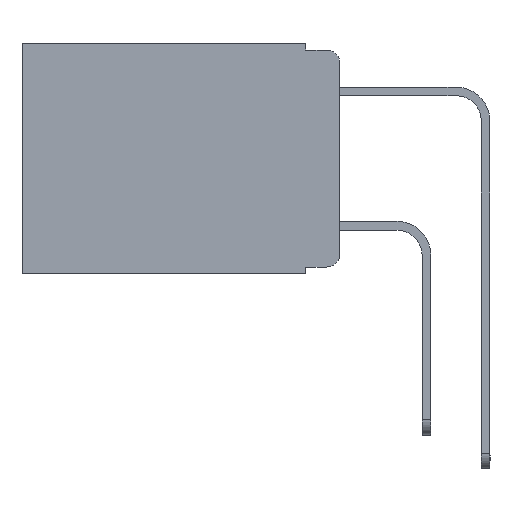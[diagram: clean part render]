
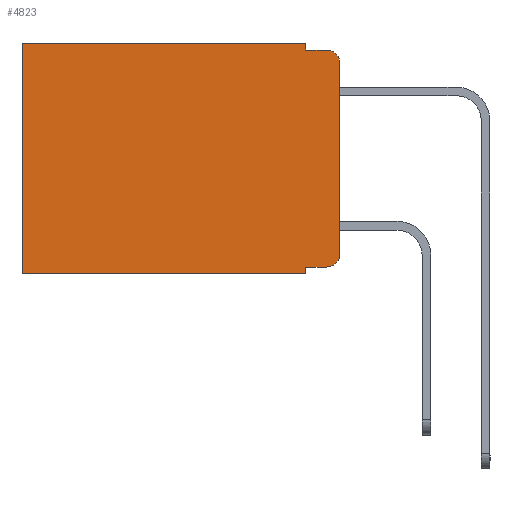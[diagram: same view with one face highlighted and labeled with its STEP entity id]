
A CAD part, left-side view. The second image highlights one B-rep face of the part: STEP entity #4823.
In plain terms, the highlighted planar face has unit normal (-1, 0, 0).
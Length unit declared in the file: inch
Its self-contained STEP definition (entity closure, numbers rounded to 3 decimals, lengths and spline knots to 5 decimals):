
#59 = ORIENTED_EDGE ( 'NONE', *, *, #6314, .F. ) ;
#996 = CARTESIAN_POINT ( 'NONE',  ( 0.298, 0.051, -0.333 ) ) ;
#1354 = EDGE_CURVE ( 'NONE', #11542, #20288, #14897, .T. ) ;
#1547 = DIRECTION ( 'NONE',  ( 1., 0., 0. ) ) ;
#1729 = VECTOR ( 'NONE', #17681, 39.37008 ) ;
#1819 = CARTESIAN_POINT ( 'NONE',  ( 0.298, 0., 0. ) ) ;
#2056 = LINE ( 'NONE', #6433, #13074 ) ;
#2120 = CARTESIAN_POINT ( 'NONE',  ( 0.298, 0.051, 0. ) ) ;
#2134 = DIRECTION ( 'NONE',  ( 0., 0., -1. ) ) ;
#2136 = CARTESIAN_POINT ( 'NONE',  ( 0.298, 0.051, -0.333 ) ) ;
#2709 = ORIENTED_EDGE ( 'NONE', *, *, #14870, .F. ) ;
#2943 = DIRECTION ( 'NONE',  ( -1., 0., 0. ) ) ;
#3644 = ORIENTED_EDGE ( 'NONE', *, *, #13271, .F. ) ;
#4561 = VERTEX_POINT ( 'NONE', #2136 ) ;
#4633 = ORIENTED_EDGE ( 'NONE', *, *, #1354, .T. ) ;
#4823 = ADVANCED_FACE ( 'NONE', ( #20280 ), #16604, .F. ) ;
#5040 = CIRCLE ( 'NONE', #22920, 0.02 ) ;
#5417 = CARTESIAN_POINT ( 'NONE',  ( 0.298, 0.051, 0. ) ) ;
#5519 = CARTESIAN_POINT ( 'NONE',  ( 0.298, 0.473, -0.343 ) ) ;
#5904 = VECTOR ( 'NONE', #26792, 39.37008 ) ;
#6314 = EDGE_CURVE ( 'NONE', #6345, #19972, #15251, .T. ) ;
#6345 = VERTEX_POINT ( 'NONE', #13186 ) ;
#6433 = CARTESIAN_POINT ( 'NONE',  ( 0.298, 0., 0. ) ) ;
#6496 = DIRECTION ( 'NONE',  ( 0., 0., -1. ) ) ;
#6515 = LINE ( 'NONE', #20582, #26492 ) ;
#6570 = CARTESIAN_POINT ( 'NONE',  ( 0.298, 0., -0.313 ) ) ;
#8101 = DIRECTION ( 'NONE',  ( 0., 0., -1. ) ) ;
#9087 = CARTESIAN_POINT ( 'NONE',  ( 0.298, 0.051, -0.01 ) ) ;
#9111 = CARTESIAN_POINT ( 'NONE',  ( 0.298, 0.02, -0.03 ) ) ;
#9128 = VECTOR ( 'NONE', #12824, 39.37008 ) ;
#9235 = VERTEX_POINT ( 'NONE', #26487 ) ;
#9357 = VECTOR ( 'NONE', #19869, 39.37008 ) ;
#9728 = VECTOR ( 'NONE', #11673, 39.37008 ) ;
#10088 = AXIS2_PLACEMENT_3D ( 'NONE', #1819, #1547, #8101 ) ;
#10370 = ORIENTED_EDGE ( 'NONE', *, *, #14620, .T. ) ;
#10512 = VERTEX_POINT ( 'NONE', #5417 ) ;
#11167 = CARTESIAN_POINT ( 'NONE',  ( 0.298, 0.473, 0. ) ) ;
#11542 = VERTEX_POINT ( 'NONE', #11167 ) ;
#11673 = DIRECTION ( 'NONE',  ( 0., 0., -1. ) ) ;
#12191 = CARTESIAN_POINT ( 'NONE',  ( 0.298, 0.02, -0.333 ) ) ;
#12503 = LINE ( 'NONE', #2120, #21305 ) ;
#12824 = DIRECTION ( 'NONE',  ( 0., 0., -1. ) ) ;
#13074 = VECTOR ( 'NONE', #25041, 39.37008 ) ;
#13186 = CARTESIAN_POINT ( 'NONE',  ( 0.298, 0.051, -0.01 ) ) ;
#13271 = EDGE_CURVE ( 'NONE', #10512, #6345, #12503, .T. ) ;
#14493 = VERTEX_POINT ( 'NONE', #12191 ) ;
#14620 = EDGE_CURVE ( 'NONE', #10512, #11542, #2056, .T. ) ;
#14870 = EDGE_CURVE ( 'NONE', #4561, #9235, #26395, .T. ) ;
#14897 = LINE ( 'NONE', #25414, #9128 ) ;
#14898 = CARTESIAN_POINT ( 'NONE',  ( 0.298, 0.02, -0.01 ) ) ;
#15251 = LINE ( 'NONE', #9087, #9357 ) ;
#15509 = EDGE_CURVE ( 'NONE', #14493, #24336, #5040, .T. ) ;
#16604 = PLANE ( 'NONE',  #10088 ) ;
#16821 = EDGE_CURVE ( 'NONE', #9235, #20288, #6515, .T. ) ;
#16909 = DIRECTION ( 'NONE',  ( -1., 0., 0. ) ) ;
#17528 = ORIENTED_EDGE ( 'NONE', *, *, #22072, .T. ) ;
#17681 = DIRECTION ( 'NONE',  ( 0., -1., 0. ) ) ;
#17815 = LINE ( 'NONE', #996, #1729 ) ;
#18314 = CARTESIAN_POINT ( 'NONE',  ( 0.298, 0.051, 0. ) ) ;
#18742 = ORIENTED_EDGE ( 'NONE', *, *, #21507, .T. ) ;
#19869 = DIRECTION ( 'NONE',  ( 0., -1., 0. ) ) ;
#19972 = VERTEX_POINT ( 'NONE', #14898 ) ;
#20280 = FACE_OUTER_BOUND ( 'NONE', #26678, .T. ) ;
#20288 = VERTEX_POINT ( 'NONE', #5519 ) ;
#20582 = CARTESIAN_POINT ( 'NONE',  ( 0.298, 0., -0.343 ) ) ;
#20673 = CARTESIAN_POINT ( 'NONE',  ( 0.298, 0., -0.03 ) ) ;
#20943 = ORIENTED_EDGE ( 'NONE', *, *, #16821, .F. ) ;
#21305 = VECTOR ( 'NONE', #6496, 39.37008 ) ;
#21507 = EDGE_CURVE ( 'NONE', #21712, #19972, #26205, .T. ) ;
#21712 = VERTEX_POINT ( 'NONE', #20673 ) ;
#21893 = ORIENTED_EDGE ( 'NONE', *, *, #15509, .T. ) ;
#22072 = EDGE_CURVE ( 'NONE', #4561, #14493, #17815, .T. ) ;
#22920 = AXIS2_PLACEMENT_3D ( 'NONE', #23059, #16909, #2134 ) ;
#23059 = CARTESIAN_POINT ( 'NONE',  ( 0.298, 0.02, -0.313 ) ) ;
#23755 = DIRECTION ( 'NONE',  ( 0., 0., -1. ) ) ;
#24014 = AXIS2_PLACEMENT_3D ( 'NONE', #9111, #2943, #23755 ) ;
#24336 = VERTEX_POINT ( 'NONE', #6570 ) ;
#24786 = CARTESIAN_POINT ( 'NONE',  ( 0.298, 0., 0. ) ) ;
#25036 = ORIENTED_EDGE ( 'NONE', *, *, #26623, .F. ) ;
#25041 = DIRECTION ( 'NONE',  ( 0., 1., 0. ) ) ;
#25109 = DIRECTION ( 'NONE',  ( 0., 1., 0. ) ) ;
#25414 = CARTESIAN_POINT ( 'NONE',  ( 0.298, 0.473, 0. ) ) ;
#26205 = CIRCLE ( 'NONE', #24014, 0.02 ) ;
#26395 = LINE ( 'NONE', #18314, #5904 ) ;
#26487 = CARTESIAN_POINT ( 'NONE',  ( 0.298, 0.051, -0.343 ) ) ;
#26492 = VECTOR ( 'NONE', #25109, 39.37008 ) ;
#26623 = EDGE_CURVE ( 'NONE', #21712, #24336, #26837, .T. ) ;
#26678 = EDGE_LOOP ( 'NONE', ( #25036, #18742, #59, #3644, #10370, #4633, #20943, #2709, #17528, #21893 ) ) ;
#26792 = DIRECTION ( 'NONE',  ( 0., 0., -1. ) ) ;
#26837 = LINE ( 'NONE', #24786, #9728 ) ;
